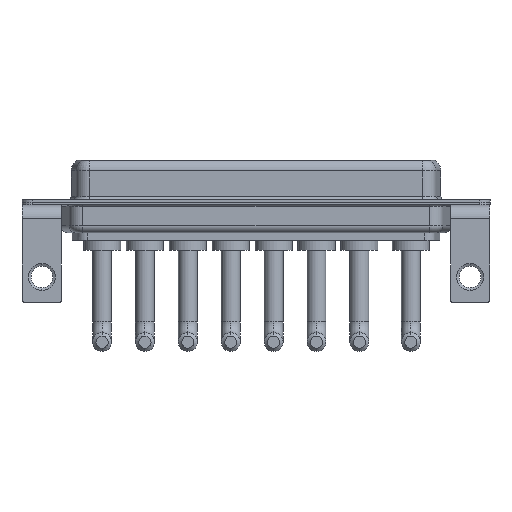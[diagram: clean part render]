
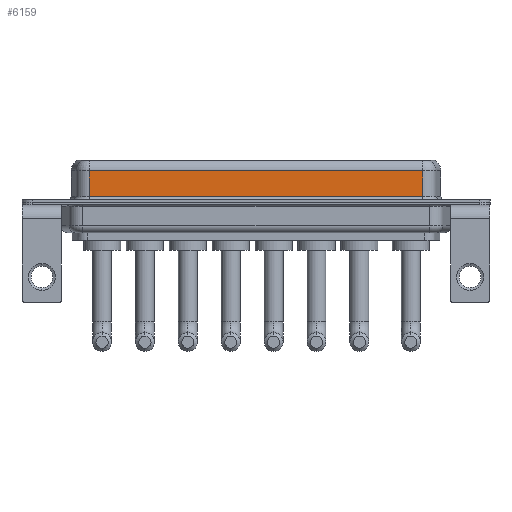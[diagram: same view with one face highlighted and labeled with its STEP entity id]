
A CAD part, front view. The second image highlights one B-rep face of the part: STEP entity #6159.
In plain terms, the highlighted planar face has unit normal (0, -1, 0).
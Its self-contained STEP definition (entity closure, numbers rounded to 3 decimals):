
#271 = AXIS2_PLACEMENT_3D ( 'NONE', #13657, #2734, #11368 ) ;
#1124 = CARTESIAN_POINT ( 'NONE',  ( 56.462, -3.95, 4.65 ) ) ;
#1452 = FACE_OUTER_BOUND ( 'NONE', #12957, .T. ) ;
#1542 = EDGE_CURVE ( 'NONE', #7875, #12223, #8995, .T. ) ;
#2491 = CARTESIAN_POINT ( 'NONE',  ( 56.462, -3.95, 4.65 ) ) ;
#2734 = DIRECTION ( 'NONE',  ( 0., 1., 0. ) ) ;
#3005 = DIRECTION ( 'NONE',  ( 1., 0., 0. ) ) ;
#3260 = VECTOR ( 'NONE', #6059, 1000. ) ;
#3484 = CARTESIAN_POINT ( 'NONE',  ( 7.038, -3.95, 4.65 ) ) ;
#3927 = LINE ( 'NONE', #6190, #3260 ) ;
#4165 = LINE ( 'NONE', #11790, #4373 ) ;
#4373 = VECTOR ( 'NONE', #3005, 1000. ) ;
#5585 = ORIENTED_EDGE ( 'NONE', *, *, #9359, .T. ) ;
#6059 = DIRECTION ( 'NONE',  ( 0., 0., -1. ) ) ;
#6137 = VERTEX_POINT ( 'NONE', #6993 ) ;
#6159 = ADVANCED_FACE ( 'NONE', ( #1452 ), #12445, .F. ) ;
#6190 = CARTESIAN_POINT ( 'NONE',  ( 7.038, -3.95, 6.4 ) ) ;
#6233 = EDGE_CURVE ( 'NONE', #6137, #13842, #4165, .T. ) ;
#6993 = CARTESIAN_POINT ( 'NONE',  ( 7.038, -3.95, 0.9 ) ) ;
#7875 = VERTEX_POINT ( 'NONE', #1124 ) ;
#8995 = LINE ( 'NONE', #2491, #10353 ) ;
#9359 = EDGE_CURVE ( 'NONE', #12223, #6137, #3927, .T. ) ;
#9670 = DIRECTION ( 'NONE',  ( 0., 0., -1. ) ) ;
#9767 = ORIENTED_EDGE ( 'NONE', *, *, #12571, .F. ) ;
#9873 = VECTOR ( 'NONE', #9670, 1000. ) ;
#10353 = VECTOR ( 'NONE', #12471, 1000. ) ;
#10371 = ORIENTED_EDGE ( 'NONE', *, *, #6233, .T. ) ;
#10434 = ORIENTED_EDGE ( 'NONE', *, *, #1542, .T. ) ;
#11072 = CARTESIAN_POINT ( 'NONE',  ( 56.462, -3.95, 0.9 ) ) ;
#11368 = DIRECTION ( 'NONE',  ( 0., 0., 1. ) ) ;
#11790 = CARTESIAN_POINT ( 'NONE',  ( 56.462, -3.95, 0.9 ) ) ;
#11867 = LINE ( 'NONE', #12017, #9873 ) ;
#12017 = CARTESIAN_POINT ( 'NONE',  ( 56.462, -3.95, 6.4 ) ) ;
#12223 = VERTEX_POINT ( 'NONE', #3484 ) ;
#12445 = PLANE ( 'NONE',  #271 ) ;
#12471 = DIRECTION ( 'NONE',  ( -1., 0., 0. ) ) ;
#12571 = EDGE_CURVE ( 'NONE', #7875, #13842, #11867, .T. ) ;
#12957 = EDGE_LOOP ( 'NONE', ( #9767, #10434, #5585, #10371 ) ) ;
#13657 = CARTESIAN_POINT ( 'NONE',  ( 56.462, -3.95, 6.4 ) ) ;
#13842 = VERTEX_POINT ( 'NONE', #11072 ) ;
